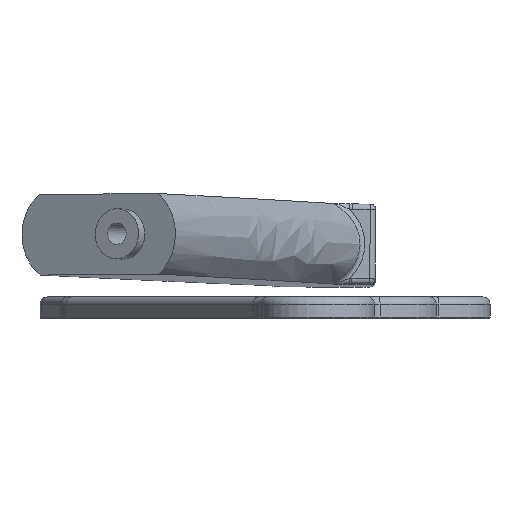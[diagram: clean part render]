
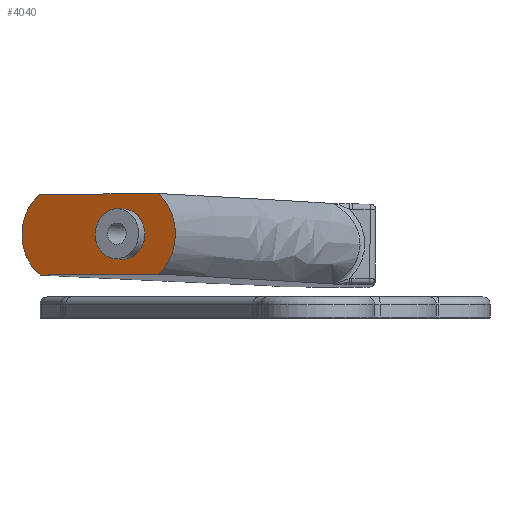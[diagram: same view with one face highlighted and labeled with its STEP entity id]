
A CAD part, front view. The second image highlights one B-rep face of the part: STEP entity #4040.
In plain terms, the highlighted planar face has unit normal (-0.5, -0.866, 0).
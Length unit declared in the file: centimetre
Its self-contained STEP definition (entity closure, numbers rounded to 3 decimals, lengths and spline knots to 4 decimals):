
#21=ELLIPSE($,#4347,0.7003,0.7);
#179=B_SPLINE_CURVE_WITH_KNOTS($,3,(#7627,#7628,#7629,#7630,#7631,#7632,
#7633,#7634,#7635,#7636,#7637,#7638,#7639,#7640),.UNSPECIFIED.,.F.,.F.,
(4,2,2,2,2,2,4),(-3.0861,-2.5385,-1.997,
-1.2773,-0.6653,-0.334,0.),
 .UNSPECIFIED.);
#183=B_SPLINE_CURVE_WITH_KNOTS($,3,(#7852,#7853,#7854,#7855,#7856,#7857,
#7858,#7859,#7860,#7861,#7862,#7863,#7864,#7865),.UNSPECIFIED.,.F.,.F.,
(4,2,2,2,2,2,4),(-2.6374,-2.2459,-1.8617,-1.3188,
-0.773,-0.3902,0.),
 .UNSPECIFIED.);
#224=LINE($,#7657,#513);
#225=LINE($,#7875,#514);
#513=VECTOR($,#5000,3.8251);
#514=VECTOR($,#5003,3.8282);
#835=FACE_BOUND($,#1187,.T.);
#918=FACE_OUTER_BOUND($,#1186,.T.);
#1186=EDGE_LOOP($,(#2942,#2943,#2944,#2945));
#1187=EDGE_LOOP($,(#2946));
#1797=VERTEX_POINT($,#7625);
#1798=VERTEX_POINT($,#7626);
#1799=VERTEX_POINT($,#7656);
#1800=VERTEX_POINT($,#7851);
#1805=VERTEX_POINT($,#7893);
#2198=EDGE_CURVE($,#1797,#1798,#179,.F.);
#2201=EDGE_CURVE($,#1798,#1799,#224,.F.);
#2203=EDGE_CURVE($,#1799,#1800,#183,.F.);
#2205=EDGE_CURVE($,#1800,#1797,#225,.T.);
#2214=EDGE_CURVE($,#1805,#1805,#21,.F.);
#2942=ORIENTED_EDGE($,*,*,#2205,.F.);
#2943=ORIENTED_EDGE($,*,*,#2203,.F.);
#2944=ORIENTED_EDGE($,*,*,#2201,.F.);
#2945=ORIENTED_EDGE($,*,*,#2198,.F.);
#2946=ORIENTED_EDGE($,*,*,#2214,.F.);
#3939=PLANE($,#4346);
#4040=ADVANCED_FACE($,(#918,#835),#3939,.F.);
#4346=AXIS2_PLACEMENT_3D($,#7892,#5020,#5021);
#4347=AXIS2_PLACEMENT_3D($,#7894,#5022,#5023);
#5000=DIRECTION($,(0.866,-0.5,0.007));
#5003=DIRECTION($,(0.866,-0.5,0.007));
#5020=DIRECTION('center_axis',(0.5,0.866,0.));
#5021=DIRECTION('ref_axis',(0.753,-0.435,-0.493));
#5022=DIRECTION('center_axis',(0.5,0.866,0.));
#5023=DIRECTION('ref_axis',(0.01,-0.006,-1.));
#7625=CARTESIAN_POINT('',(-23.5819,-0.2408,2.1396));
#7626=CARTESIAN_POINT('',(-23.5667,-0.2496,-0.1091));
#7627=CARTESIAN_POINT('Ctrl Pts',(-23.5667,-0.2496,
-0.1091));
#7628=CARTESIAN_POINT('Ctrl Pts',(-23.4771,-0.3013,
-0.0254));
#7629=CARTESIAN_POINT('Ctrl Pts',(-23.3976,-0.3472,
0.0726));
#7630=CARTESIAN_POINT('Ctrl Pts',(-23.2651,-0.4237,
0.2905));
#7631=CARTESIAN_POINT('Ctrl Pts',(-23.2123,-0.4542,
0.4093));
#7632=CARTESIAN_POINT('Ctrl Pts',(-23.1243,-0.505,0.7003));
#7633=CARTESIAN_POINT('Ctrl Pts',(-23.0974,-0.5205,
0.8872));
#7634=CARTESIAN_POINT('Ctrl Pts',(-23.1144,-0.5107,1.2534));
#7635=CARTESIAN_POINT('Ctrl Pts',(-23.1487,-0.4909,
1.439));
#7636=CARTESIAN_POINT('Ctrl Pts',(-23.2656,-0.4234,
1.7239));
#7637=CARTESIAN_POINT('Ctrl Pts',(-23.3167,-0.3939,
1.8184));
#7638=CARTESIAN_POINT('Ctrl Pts',(-23.4369,-0.3245,
1.9922));
#7639=CARTESIAN_POINT('Ctrl Pts',(-23.506,-0.2846,
2.071));
#7640=CARTESIAN_POINT('Ctrl Pts',(-23.5819,-0.2408,2.1396));
#7656=CARTESIAN_POINT('',(-26.8793,1.663,-0.1378));
#7657=CARTESIAN_POINT($,(-25.3657,0.7891,-0.1247));
#7851=CARTESIAN_POINT('',(-26.8972,1.6733,2.1109));
#7852=CARTESIAN_POINT('Ctrl Pts',(-26.8972,1.6733,2.1109));
#7853=CARTESIAN_POINT('Ctrl Pts',(-26.9888,1.7262,2.0345));
#7854=CARTESIAN_POINT('Ctrl Pts',(-27.0707,1.7735,1.943));
#7855=CARTESIAN_POINT('Ctrl Pts',(-27.2077,1.8526,1.7386));
#7856=CARTESIAN_POINT('Ctrl Pts',(-27.2629,1.8844,1.6268));
#7857=CARTESIAN_POINT('Ctrl Pts',(-27.3617,1.9415,1.3405));
#7858=CARTESIAN_POINT('Ctrl Pts',(-27.3904,1.9581,1.1612));
#7859=CARTESIAN_POINT('Ctrl Pts',(-27.3871,1.9562,0.8008));
#7860=CARTESIAN_POINT('Ctrl Pts',(-27.355,1.9376,0.622));
#7861=CARTESIAN_POINT('Ctrl Pts',(-27.2508,1.8774,0.3377));
#7862=CARTESIAN_POINT('Ctrl Pts',(-27.1939,1.8446,0.2275));
#7863=CARTESIAN_POINT('Ctrl Pts',(-27.0543,1.764,0.0267));
#7864=CARTESIAN_POINT('Ctrl Pts',(-26.9715,1.7162,-0.0631));
#7865=CARTESIAN_POINT('Ctrl Pts',(-26.8793,1.663,-0.1378));
#7875=CARTESIAN_POINT($,(-24.6061,0.3505,2.1307));
#7892=CARTESIAN_POINT('Origin',(-24.9679,0.5594,0.9613));
#7893=CARTESIAN_POINT('',(-24.5751,0.3326,1.7069));
#7894=CARTESIAN_POINT('Origin',(-24.568,0.3285,1.0066));
